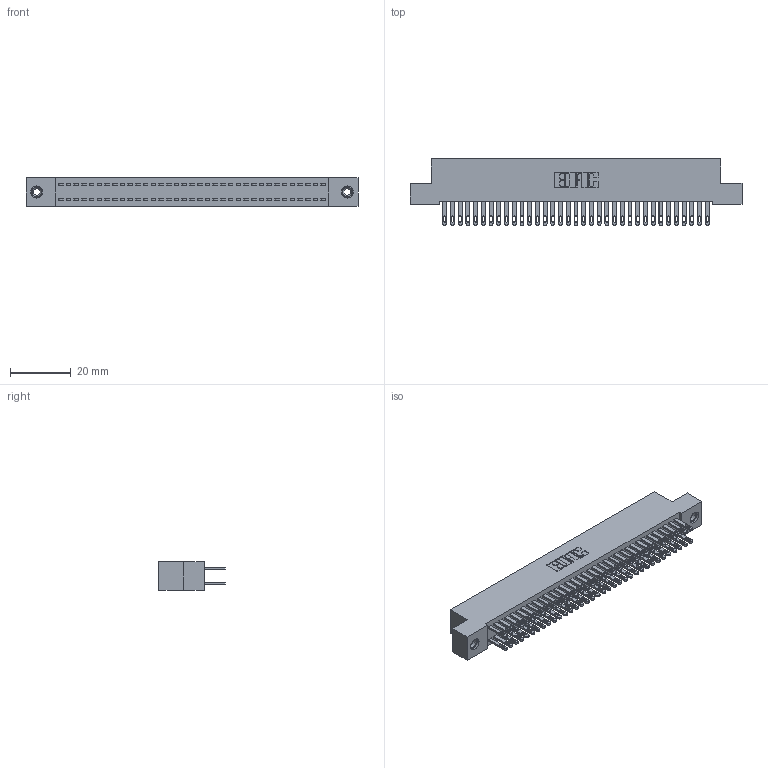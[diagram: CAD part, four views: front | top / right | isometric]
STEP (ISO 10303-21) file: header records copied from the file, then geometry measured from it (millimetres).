
FILE_DESCRIPTION (( 'STEP AP203' ), '1' );
FILE_NAME ('892-070-500-208.STEP', '2020-09-21T19:42:05', ( '' ), ( '' ), 'SwSTEP 2.0', 'SolidWorks 2020', '' );
FILE_SCHEMA (( 'CONFIG_CONTROL_DESIGN' ));
Length unit declared in the file: inch
Products named in the file (4): 842 Part_TI; 345-292-001_345-293-100; 345-250-001_345-250-003-102; 892-070-500-208
Assembly tree (73 placements, depth 2):
  892-070-500-208
    842 Part_TI
    345-292-001_345-293-100  x70
    345-250-001_345-250-003-102  x2
Bounding box: 109.22 x 21.85 x 9.4 mm (x, y, z)
Volume: 9988.5 mm3; surface area: 16766.8 mm2
Topology: 73 solids, 73 shells, 3530 faces, 10725 edges, 7142 vertices
Faces by surface type: plane 2198, cylinder 1316, cone 12, torus 4
Entity records: 24406 total; most frequent: CARTESIAN_POINT 4033, ORIENTED_EDGE 3962, DIRECTION 3491, EDGE_CURVE 1981, LINE 1829, VECTOR 1829, VERTEX_POINT 1316, AXIS2_PLACEMENT_3D 831
